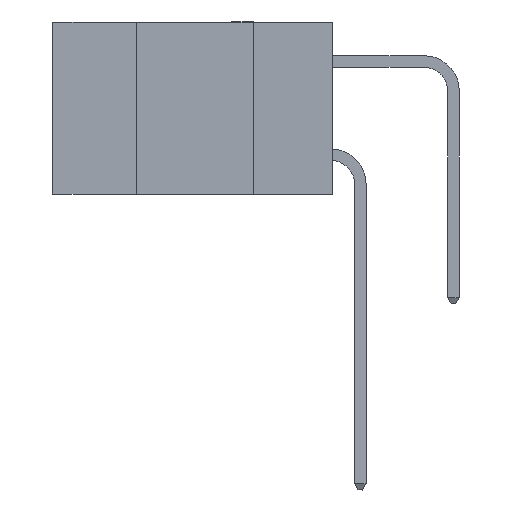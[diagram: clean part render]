
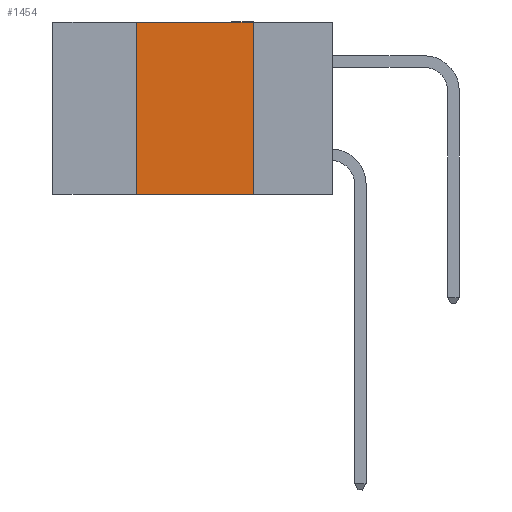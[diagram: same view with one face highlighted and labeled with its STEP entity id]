
A CAD part, left-side view. The second image highlights one B-rep face of the part: STEP entity #1454.
In plain terms, the highlighted planar face has unit normal (-1, 0, 0).
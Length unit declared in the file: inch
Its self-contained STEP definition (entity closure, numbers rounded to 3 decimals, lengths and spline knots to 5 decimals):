
#479 = CARTESIAN_POINT ( 'NONE',  ( 0., 0.42, 0. ) ) ;
#875 = DIRECTION ( 'NONE',  ( 0., -1., 0. ) ) ;
#1242 = DIRECTION ( 'NONE',  ( 0., 0., -1. ) ) ;
#1370 = CARTESIAN_POINT ( 'NONE',  ( 0., 0.6, 0. ) ) ;
#1426 = LINE ( 'NONE', #479, #7465 ) ;
#1454 = ADVANCED_FACE ( 'NONE', ( #6740 ), #1505, .F. ) ;
#1505 = PLANE ( 'NONE',  #2287 ) ;
#2028 = ORIENTED_EDGE ( 'NONE', *, *, #12202, .F. ) ;
#2287 = AXIS2_PLACEMENT_3D ( 'NONE', #1370, #11610, #4471 ) ;
#2591 = ORIENTED_EDGE ( 'NONE', *, *, #7844, .F. ) ;
#2866 = VERTEX_POINT ( 'NONE', #8007 ) ;
#2995 = EDGE_CURVE ( 'NONE', #12819, #6401, #4458, .T. ) ;
#3318 = EDGE_CURVE ( 'NONE', #2866, #4773, #12278, .T. ) ;
#3333 = VECTOR ( 'NONE', #3880, 39.37008 ) ;
#3754 = CARTESIAN_POINT ( 'NONE',  ( 0., 0.42, 0. ) ) ;
#3880 = DIRECTION ( 'NONE',  ( 0., -1., 0. ) ) ;
#4458 = LINE ( 'NONE', #13083, #5743 ) ;
#4471 = DIRECTION ( 'NONE',  ( 0., 0., -1. ) ) ;
#4773 = VERTEX_POINT ( 'NONE', #6827 ) ;
#5743 = VECTOR ( 'NONE', #875, 39.37008 ) ;
#6401 = VERTEX_POINT ( 'NONE', #10512 ) ;
#6740 = FACE_OUTER_BOUND ( 'NONE', #9773, .T. ) ;
#6827 = CARTESIAN_POINT ( 'NONE',  ( 0., 0.17, -0.37 ) ) ;
#7465 = VECTOR ( 'NONE', #8644, 39.37008 ) ;
#7844 = EDGE_CURVE ( 'NONE', #6401, #4773, #10609, .T. ) ;
#7872 = VECTOR ( 'NONE', #1242, 39.37008 ) ;
#8007 = CARTESIAN_POINT ( 'NONE',  ( 0., 0.42, -0.37 ) ) ;
#8644 = DIRECTION ( 'NONE',  ( 0., 0., 1. ) ) ;
#9493 = CARTESIAN_POINT ( 'NONE',  ( 0., 0.17, 0. ) ) ;
#9773 = EDGE_LOOP ( 'NONE', ( #2591, #12744, #2028, #12855 ) ) ;
#10512 = CARTESIAN_POINT ( 'NONE',  ( 0., 0.17, 0. ) ) ;
#10609 = LINE ( 'NONE', #9493, #7872 ) ;
#11610 = DIRECTION ( 'NONE',  ( 1., 0., 0. ) ) ;
#12088 = CARTESIAN_POINT ( 'NONE',  ( 0., 0.6, -0.37 ) ) ;
#12202 = EDGE_CURVE ( 'NONE', #2866, #12819, #1426, .T. ) ;
#12278 = LINE ( 'NONE', #12088, #3333 ) ;
#12744 = ORIENTED_EDGE ( 'NONE', *, *, #2995, .F. ) ;
#12819 = VERTEX_POINT ( 'NONE', #3754 ) ;
#12855 = ORIENTED_EDGE ( 'NONE', *, *, #3318, .T. ) ;
#13083 = CARTESIAN_POINT ( 'NONE',  ( 0., 0.6, 0. ) ) ;
